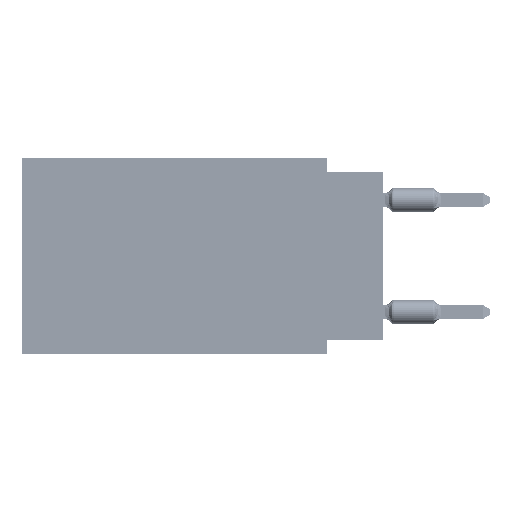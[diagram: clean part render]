
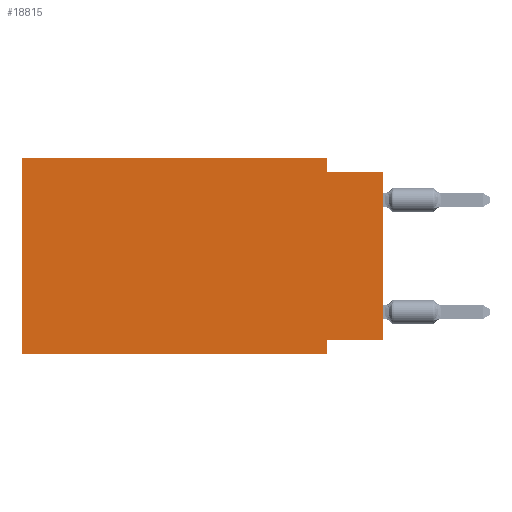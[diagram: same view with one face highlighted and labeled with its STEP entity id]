
A CAD part, left-side view. The second image highlights one B-rep face of the part: STEP entity #18815.
In plain terms, the highlighted planar face has unit normal (-1, 0, 0).
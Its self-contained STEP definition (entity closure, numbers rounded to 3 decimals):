
#1299 = VECTOR ( 'NONE', #48706, 1000. ) ;
#2112 = LINE ( 'NONE', #60296, #64450 ) ;
#4325 = VECTOR ( 'NONE', #16142, 1000. ) ;
#5761 = DIRECTION ( 'NONE',  ( 0., -1., 0. ) ) ;
#8519 = LINE ( 'NONE', #30916, #4325 ) ;
#9839 = ORIENTED_EDGE ( 'NONE', *, *, #49189, .F. ) ;
#10370 = EDGE_CURVE ( 'NONE', #42558, #90141, #2112, .T. ) ;
#12117 = CARTESIAN_POINT ( 'NONE',  ( 0., 0., -8.255 ) ) ;
#15570 = ORIENTED_EDGE ( 'NONE', *, *, #30521, .F. ) ;
#16142 = DIRECTION ( 'NONE',  ( 0., 0., -1. ) ) ;
#16899 = VERTEX_POINT ( 'NONE', #65155 ) ;
#18218 = EDGE_CURVE ( 'NONE', #77257, #91661, #77413, .T. ) ;
#18765 = CARTESIAN_POINT ( 'NONE',  ( 0., 16.383, -8.89 ) ) ;
#18815 = ADVANCED_FACE ( 'NONE', ( #45296 ), #53410, .F. ) ;
#19490 = VERTEX_POINT ( 'NONE', #72617 ) ;
#20653 = VECTOR ( 'NONE', #36376, 1000. ) ;
#21386 = EDGE_CURVE ( 'NONE', #19490, #63248, #42005, .T. ) ;
#22284 = VECTOR ( 'NONE', #29374, 1000. ) ;
#24088 = DIRECTION ( 'NONE',  ( 0., -1., 0. ) ) ;
#24775 = EDGE_LOOP ( 'NONE', ( #27862, #39026, #15570, #92794, #9839, #31117, #44941, #49556 ) ) ;
#27862 = ORIENTED_EDGE ( 'NONE', *, *, #61901, .T. ) ;
#28478 = DIRECTION ( 'NONE',  ( 0., 0., -1. ) ) ;
#29374 = DIRECTION ( 'NONE',  ( 0., 0., 1. ) ) ;
#30173 = DIRECTION ( 'NONE',  ( 0., 0., 1. ) ) ;
#30521 = EDGE_CURVE ( 'NONE', #63248, #42558, #63782, .T. ) ;
#30916 = CARTESIAN_POINT ( 'NONE',  ( 0., 2.54, -8.89 ) ) ;
#31117 = ORIENTED_EDGE ( 'NONE', *, *, #91161, .T. ) ;
#36376 = DIRECTION ( 'NONE',  ( 0., 1., 0. ) ) ;
#36533 = CARTESIAN_POINT ( 'NONE',  ( 0., 0., 0. ) ) ;
#37790 = LINE ( 'NONE', #66367, #51019 ) ;
#39026 = ORIENTED_EDGE ( 'NONE', *, *, #10370, .F. ) ;
#40990 = EDGE_CURVE ( 'NONE', #91661, #16899, #8519, .T. ) ;
#42005 = LINE ( 'NONE', #71070, #43789 ) ;
#42558 = VERTEX_POINT ( 'NONE', #50208 ) ;
#42710 = CARTESIAN_POINT ( 'NONE',  ( 0., 0., -8.255 ) ) ;
#43789 = VECTOR ( 'NONE', #5761, 1000. ) ;
#44799 = CARTESIAN_POINT ( 'NONE',  ( 0., 0., -0.635 ) ) ;
#44941 = ORIENTED_EDGE ( 'NONE', *, *, #40990, .F. ) ;
#45296 = FACE_OUTER_BOUND ( 'NONE', #24775, .T. ) ;
#48153 = AXIS2_PLACEMENT_3D ( 'NONE', #81993, #75316, #74385 ) ;
#48706 = DIRECTION ( 'NONE',  ( 0., -1., 0. ) ) ;
#49189 = EDGE_CURVE ( 'NONE', #76238, #19490, #37790, .T. ) ;
#49556 = ORIENTED_EDGE ( 'NONE', *, *, #18218, .F. ) ;
#50208 = CARTESIAN_POINT ( 'NONE',  ( 0., 2.54, -0.635 ) ) ;
#51019 = VECTOR ( 'NONE', #30173, 1000. ) ;
#53410 = PLANE ( 'NONE',  #48153 ) ;
#57128 = CARTESIAN_POINT ( 'NONE',  ( 0., 2.54, -8.255 ) ) ;
#60296 = CARTESIAN_POINT ( 'NONE',  ( 0., 0., -0.635 ) ) ;
#61901 = EDGE_CURVE ( 'NONE', #77257, #90141, #64661, .T. ) ;
#63248 = VERTEX_POINT ( 'NONE', #82750 ) ;
#63782 = LINE ( 'NONE', #77603, #78912 ) ;
#64450 = VECTOR ( 'NONE', #24088, 1000. ) ;
#64661 = LINE ( 'NONE', #36533, #22284 ) ;
#65155 = CARTESIAN_POINT ( 'NONE',  ( 0., 2.54, -8.89 ) ) ;
#66367 = CARTESIAN_POINT ( 'NONE',  ( 0., 16.383, 0. ) ) ;
#70603 = LINE ( 'NONE', #93455, #1299 ) ;
#71070 = CARTESIAN_POINT ( 'NONE',  ( 0., 16.383, 0. ) ) ;
#72617 = CARTESIAN_POINT ( 'NONE',  ( 0., 16.383, 0. ) ) ;
#74385 = DIRECTION ( 'NONE',  ( 0., 0., -1. ) ) ;
#75316 = DIRECTION ( 'NONE',  ( 1., 0., 0. ) ) ;
#76238 = VERTEX_POINT ( 'NONE', #18765 ) ;
#77257 = VERTEX_POINT ( 'NONE', #42710 ) ;
#77413 = LINE ( 'NONE', #12117, #20653 ) ;
#77603 = CARTESIAN_POINT ( 'NONE',  ( 0., 2.54, 0. ) ) ;
#78912 = VECTOR ( 'NONE', #28478, 1000. ) ;
#81993 = CARTESIAN_POINT ( 'NONE',  ( 0., 16.383, 0. ) ) ;
#82750 = CARTESIAN_POINT ( 'NONE',  ( 0., 2.54, 0. ) ) ;
#90141 = VERTEX_POINT ( 'NONE', #44799 ) ;
#91161 = EDGE_CURVE ( 'NONE', #76238, #16899, #70603, .T. ) ;
#91661 = VERTEX_POINT ( 'NONE', #57128 ) ;
#92794 = ORIENTED_EDGE ( 'NONE', *, *, #21386, .F. ) ;
#93455 = CARTESIAN_POINT ( 'NONE',  ( 0., 16.383, -8.89 ) ) ;
